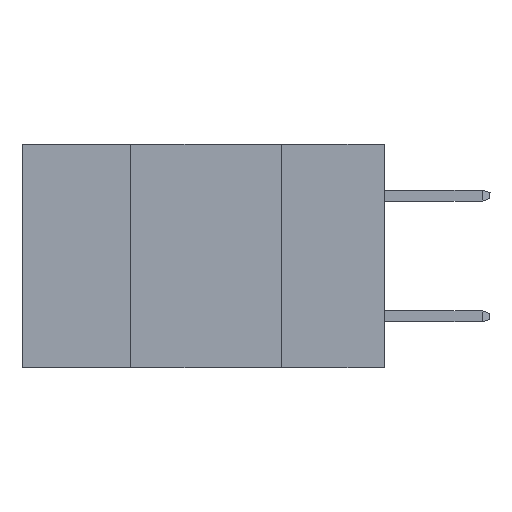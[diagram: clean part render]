
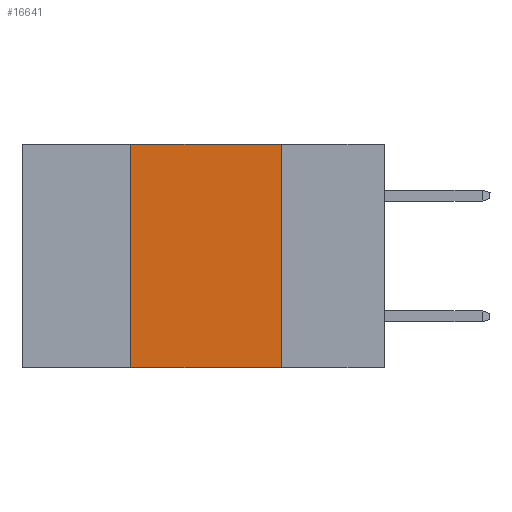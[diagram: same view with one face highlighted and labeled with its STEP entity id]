
A CAD part, left-side view. The second image highlights one B-rep face of the part: STEP entity #16641.
In plain terms, the highlighted planar face has unit normal (-1, 0, 0).
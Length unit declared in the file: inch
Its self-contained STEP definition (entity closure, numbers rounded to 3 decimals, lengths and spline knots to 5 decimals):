
#152 = DIRECTION ( 'NONE',  ( 1., 0., 0. ) ) ;
#269 = DIRECTION ( 'NONE',  ( 0., 0., 1. ) ) ;
#2032 = EDGE_CURVE ( 'NONE', #10914, #18999, #14773, .T. ) ;
#2811 = CARTESIAN_POINT ( 'NONE',  ( 0., 0.6, -0.37 ) ) ;
#4181 = LINE ( 'NONE', #9050, #8118 ) ;
#4734 = VERTEX_POINT ( 'NONE', #11525 ) ;
#4792 = PLANE ( 'NONE',  #8009 ) ;
#5408 = EDGE_CURVE ( 'NONE', #18999, #16188, #6152, .T. ) ;
#6152 = LINE ( 'NONE', #11441, #6631 ) ;
#6631 = VECTOR ( 'NONE', #17158, 39.37008 ) ;
#8008 = VECTOR ( 'NONE', #269, 39.37008 ) ;
#8009 = AXIS2_PLACEMENT_3D ( 'NONE', #12928, #152, #12855 ) ;
#8118 = VECTOR ( 'NONE', #18468, 39.37008 ) ;
#8624 = ORIENTED_EDGE ( 'NONE', *, *, #5408, .F. ) ;
#9050 = CARTESIAN_POINT ( 'NONE',  ( 0., 0.17, 0. ) ) ;
#9767 = CARTESIAN_POINT ( 'NONE',  ( 0., 0.42, 0. ) ) ;
#10035 = LINE ( 'NONE', #2811, #17485 ) ;
#10914 = VERTEX_POINT ( 'NONE', #14390 ) ;
#11441 = CARTESIAN_POINT ( 'NONE',  ( 0., 0.6, 0. ) ) ;
#11525 = CARTESIAN_POINT ( 'NONE',  ( 0., 0.17, -0.37 ) ) ;
#12365 = DIRECTION ( 'NONE',  ( 0., -1., 0. ) ) ;
#12812 = EDGE_LOOP ( 'NONE', ( #15122, #8624, #18201, #15024 ) ) ;
#12855 = DIRECTION ( 'NONE',  ( 0., 0., -1. ) ) ;
#12928 = CARTESIAN_POINT ( 'NONE',  ( 0., 0.6, 0. ) ) ;
#14102 = CARTESIAN_POINT ( 'NONE',  ( 0., 0.17, 0. ) ) ;
#14390 = CARTESIAN_POINT ( 'NONE',  ( 0., 0.42, -0.37 ) ) ;
#14773 = LINE ( 'NONE', #9767, #8008 ) ;
#15024 = ORIENTED_EDGE ( 'NONE', *, *, #17850, .T. ) ;
#15074 = EDGE_CURVE ( 'NONE', #16188, #4734, #4181, .T. ) ;
#15122 = ORIENTED_EDGE ( 'NONE', *, *, #15074, .F. ) ;
#16188 = VERTEX_POINT ( 'NONE', #14102 ) ;
#16641 = ADVANCED_FACE ( 'NONE', ( #19007 ), #4792, .F. ) ;
#17158 = DIRECTION ( 'NONE',  ( 0., -1., 0. ) ) ;
#17485 = VECTOR ( 'NONE', #12365, 39.37008 ) ;
#17850 = EDGE_CURVE ( 'NONE', #10914, #4734, #10035, .T. ) ;
#18201 = ORIENTED_EDGE ( 'NONE', *, *, #2032, .F. ) ;
#18468 = DIRECTION ( 'NONE',  ( 0., 0., -1. ) ) ;
#18999 = VERTEX_POINT ( 'NONE', #19404 ) ;
#19007 = FACE_OUTER_BOUND ( 'NONE', #12812, .T. ) ;
#19404 = CARTESIAN_POINT ( 'NONE',  ( 0., 0.42, 0. ) ) ;
